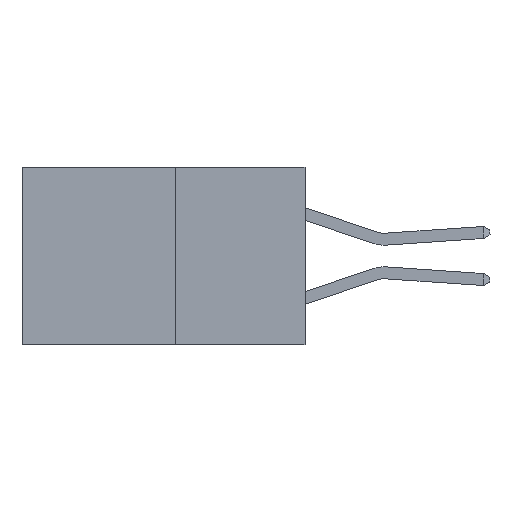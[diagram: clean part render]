
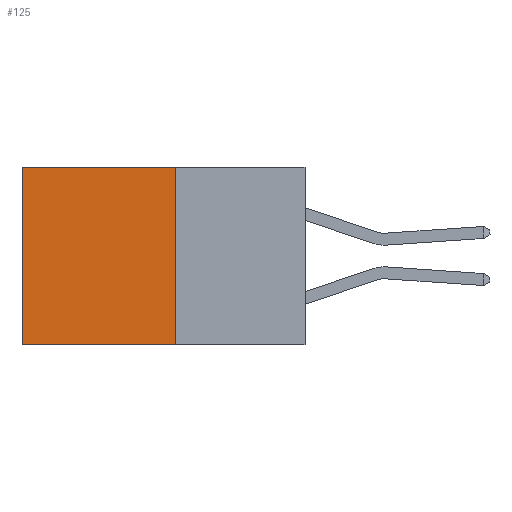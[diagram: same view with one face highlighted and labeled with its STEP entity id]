
A CAD part, left-side view. The second image highlights one B-rep face of the part: STEP entity #125.
In plain terms, the highlighted planar face has unit normal (-1, 0, 0).
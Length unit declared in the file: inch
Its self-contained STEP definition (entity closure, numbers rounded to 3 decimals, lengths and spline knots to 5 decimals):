
#125 = ADVANCED_FACE ( 'NONE', ( #16172 ), #6300, .F. ) ;
#369 = VECTOR ( 'NONE', #19614, 39.37008 ) ;
#675 = DIRECTION ( 'NONE',  ( 0., 1., 0. ) ) ;
#2004 = VERTEX_POINT ( 'NONE', #5161 ) ;
#2708 = ORIENTED_EDGE ( 'NONE', *, *, #15499, .T. ) ;
#3087 = LINE ( 'NONE', #21574, #12869 ) ;
#3965 = CARTESIAN_POINT ( 'NONE',  ( 0.277, 0.27, -0.37 ) ) ;
#4553 = LINE ( 'NONE', #3965, #369 ) ;
#5161 = CARTESIAN_POINT ( 'NONE',  ( 0.277, 0.59, 0. ) ) ;
#5926 = DIRECTION ( 'NONE',  ( 0., 1., 0. ) ) ;
#6300 = PLANE ( 'NONE',  #9525 ) ;
#7078 = LINE ( 'NONE', #21284, #18195 ) ;
#7444 = EDGE_CURVE ( 'NONE', #2004, #7892, #7078, .T. ) ;
#7522 = VECTOR ( 'NONE', #5926, 39.37008 ) ;
#7892 = VERTEX_POINT ( 'NONE', #8567 ) ;
#8129 = EDGE_CURVE ( 'NONE', #11857, #21805, #4553, .T. ) ;
#8321 = DIRECTION ( 'NONE',  ( 1., 0., 0. ) ) ;
#8540 = CARTESIAN_POINT ( 'NONE',  ( 0.277, 0.27, -0.37 ) ) ;
#8567 = CARTESIAN_POINT ( 'NONE',  ( 0.277, 0.59, -0.37 ) ) ;
#8840 = ORIENTED_EDGE ( 'NONE', *, *, #8129, .F. ) ;
#9525 = AXIS2_PLACEMENT_3D ( 'NONE', #8540, #8321, #9971 ) ;
#9971 = DIRECTION ( 'NONE',  ( 0., 0., -1. ) ) ;
#11857 = VERTEX_POINT ( 'NONE', #15136 ) ;
#12564 = DIRECTION ( 'NONE',  ( 0., 0., -1. ) ) ;
#12869 = VECTOR ( 'NONE', #675, 39.37008 ) ;
#14547 = CARTESIAN_POINT ( 'NONE',  ( 0.277, 0.27, 0. ) ) ;
#14969 = EDGE_CURVE ( 'NONE', #21805, #7892, #3087, .T. ) ;
#15136 = CARTESIAN_POINT ( 'NONE',  ( 0.277, 0.27, 0. ) ) ;
#15499 = EDGE_CURVE ( 'NONE', #11857, #2004, #21315, .T. ) ;
#16172 = FACE_OUTER_BOUND ( 'NONE', #17398, .T. ) ;
#17398 = EDGE_LOOP ( 'NONE', ( #19217, #19949, #8840, #2708 ) ) ;
#17556 = CARTESIAN_POINT ( 'NONE',  ( 0.277, 0.27, -0.37 ) ) ;
#18195 = VECTOR ( 'NONE', #12564, 39.37008 ) ;
#19217 = ORIENTED_EDGE ( 'NONE', *, *, #7444, .T. ) ;
#19614 = DIRECTION ( 'NONE',  ( 0., 0., -1. ) ) ;
#19949 = ORIENTED_EDGE ( 'NONE', *, *, #14969, .F. ) ;
#21284 = CARTESIAN_POINT ( 'NONE',  ( 0.277, 0.59, -0.37 ) ) ;
#21315 = LINE ( 'NONE', #14547, #7522 ) ;
#21574 = CARTESIAN_POINT ( 'NONE',  ( 0.277, 0.27, -0.37 ) ) ;
#21805 = VERTEX_POINT ( 'NONE', #17556 ) ;
